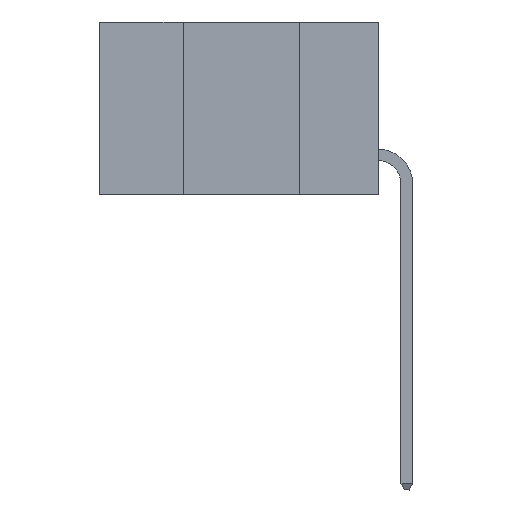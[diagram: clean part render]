
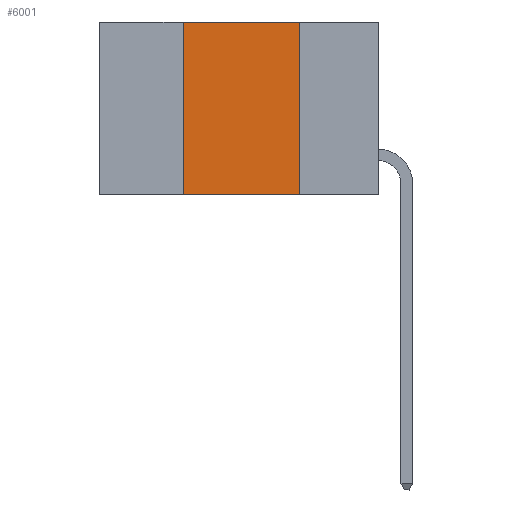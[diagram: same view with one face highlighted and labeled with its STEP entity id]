
A CAD part, left-side view. The second image highlights one B-rep face of the part: STEP entity #6001.
In plain terms, the highlighted planar face has unit normal (-1, 0, 0).
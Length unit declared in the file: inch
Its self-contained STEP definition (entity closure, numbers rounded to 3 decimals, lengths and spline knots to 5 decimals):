
#312 = CARTESIAN_POINT ( 'NONE',  ( 0., 0.42, -0.37 ) ) ;
#362 = VECTOR ( 'NONE', #5263, 39.37008 ) ;
#1300 = ORIENTED_EDGE ( 'NONE', *, *, #5317, .F. ) ;
#1884 = VERTEX_POINT ( 'NONE', #3137 ) ;
#1940 = ORIENTED_EDGE ( 'NONE', *, *, #8387, .T. ) ;
#2244 = DIRECTION ( 'NONE',  ( 0., 0., 1. ) ) ;
#3048 = CARTESIAN_POINT ( 'NONE',  ( 0., 0.17, -0.37 ) ) ;
#3122 = VECTOR ( 'NONE', #9443, 39.37008 ) ;
#3137 = CARTESIAN_POINT ( 'NONE',  ( 0., 0.42, -0.37 ) ) ;
#3635 = CARTESIAN_POINT ( 'NONE',  ( 0., 0.42, 0. ) ) ;
#4203 = CARTESIAN_POINT ( 'NONE',  ( 0., 0.6, 0. ) ) ;
#4297 = LINE ( 'NONE', #312, #10651 ) ;
#4753 = LINE ( 'NONE', #10937, #9693 ) ;
#5069 = FACE_OUTER_BOUND ( 'NONE', #10145, .T. ) ;
#5129 = DIRECTION ( 'NONE',  ( 1., 0., 0. ) ) ;
#5263 = DIRECTION ( 'NONE',  ( 0., -1., 0. ) ) ;
#5317 = EDGE_CURVE ( 'NONE', #11796, #6326, #4753, .T. ) ;
#5635 = ORIENTED_EDGE ( 'NONE', *, *, #10437, .F. ) ;
#5957 = DIRECTION ( 'NONE',  ( 0., 0., -1. ) ) ;
#6001 = ADVANCED_FACE ( 'NONE', ( #5069 ), #6138, .F. ) ;
#6138 = PLANE ( 'NONE',  #9491 ) ;
#6326 = VERTEX_POINT ( 'NONE', #3048 ) ;
#7102 = VERTEX_POINT ( 'NONE', #3635 ) ;
#7192 = EDGE_CURVE ( 'NONE', #7102, #11796, #11239, .T. ) ;
#7743 = CARTESIAN_POINT ( 'NONE',  ( 0., 0.17, 0. ) ) ;
#8170 = LINE ( 'NONE', #8363, #3122 ) ;
#8363 = CARTESIAN_POINT ( 'NONE',  ( 0., 0.6, -0.37 ) ) ;
#8387 = EDGE_CURVE ( 'NONE', #1884, #6326, #8170, .T. ) ;
#9173 = DIRECTION ( 'NONE',  ( 0., 0., -1. ) ) ;
#9443 = DIRECTION ( 'NONE',  ( 0., -1., 0. ) ) ;
#9491 = AXIS2_PLACEMENT_3D ( 'NONE', #10175, #5129, #9173 ) ;
#9693 = VECTOR ( 'NONE', #5957, 39.37008 ) ;
#10145 = EDGE_LOOP ( 'NONE', ( #1300, #11817, #5635, #1940 ) ) ;
#10175 = CARTESIAN_POINT ( 'NONE',  ( 0., 0.6, 0. ) ) ;
#10437 = EDGE_CURVE ( 'NONE', #1884, #7102, #4297, .T. ) ;
#10651 = VECTOR ( 'NONE', #2244, 39.37008 ) ;
#10937 = CARTESIAN_POINT ( 'NONE',  ( 0., 0.17, -0.37 ) ) ;
#11239 = LINE ( 'NONE', #4203, #362 ) ;
#11796 = VERTEX_POINT ( 'NONE', #7743 ) ;
#11817 = ORIENTED_EDGE ( 'NONE', *, *, #7192, .F. ) ;
